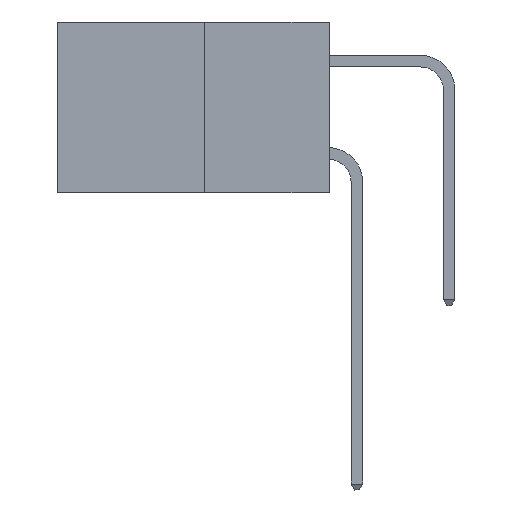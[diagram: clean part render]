
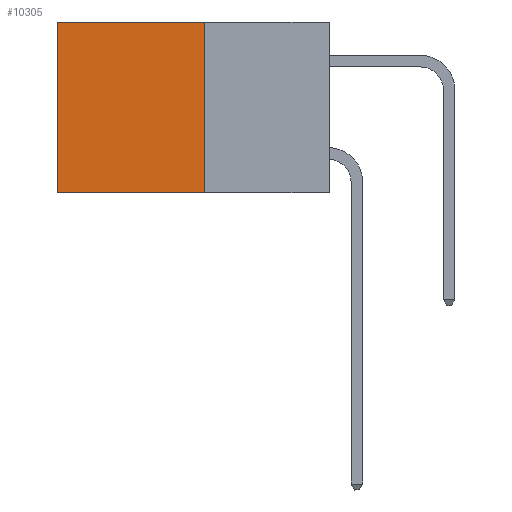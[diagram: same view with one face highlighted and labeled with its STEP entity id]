
A CAD part, left-side view. The second image highlights one B-rep face of the part: STEP entity #10305.
In plain terms, the highlighted planar face has unit normal (-1, 0, 0).
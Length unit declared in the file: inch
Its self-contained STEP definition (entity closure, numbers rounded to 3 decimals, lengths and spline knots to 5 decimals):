
#255 = LINE ( 'NONE', #12976, #3978 ) ;
#1018 = PLANE ( 'NONE',  #6401 ) ;
#1165 = EDGE_CURVE ( 'NONE', #4033, #9187, #13023, .T. ) ;
#1193 = CARTESIAN_POINT ( 'NONE',  ( 0.277, 0.59, 0. ) ) ;
#2083 = FACE_OUTER_BOUND ( 'NONE', #4950, .T. ) ;
#2296 = DIRECTION ( 'NONE',  ( 1., 0., 0. ) ) ;
#3022 = EDGE_CURVE ( 'NONE', #4033, #8451, #11666, .T. ) ;
#3113 = VECTOR ( 'NONE', #9914, 39.37008 ) ;
#3680 = CARTESIAN_POINT ( 'NONE',  ( 0.277, 0.27, 0. ) ) ;
#3850 = DIRECTION ( 'NONE',  ( 0., 1., 0. ) ) ;
#3978 = VECTOR ( 'NONE', #14117, 39.37008 ) ;
#4033 = VERTEX_POINT ( 'NONE', #3680 ) ;
#4950 = EDGE_LOOP ( 'NONE', ( #5924, #10772, #14763, #9836 ) ) ;
#5924 = ORIENTED_EDGE ( 'NONE', *, *, #13153, .T. ) ;
#6401 = AXIS2_PLACEMENT_3D ( 'NONE', #9809, #2296, #11016 ) ;
#8451 = VERTEX_POINT ( 'NONE', #1193 ) ;
#8939 = VECTOR ( 'NONE', #3850, 39.37008 ) ;
#8969 = CARTESIAN_POINT ( 'NONE',  ( 0.277, 0.27, -0.37 ) ) ;
#9187 = VERTEX_POINT ( 'NONE', #8969 ) ;
#9809 = CARTESIAN_POINT ( 'NONE',  ( 0.277, 0.27, -0.37 ) ) ;
#9836 = ORIENTED_EDGE ( 'NONE', *, *, #3022, .T. ) ;
#9914 = DIRECTION ( 'NONE',  ( 0., 0., -1. ) ) ;
#10180 = CARTESIAN_POINT ( 'NONE',  ( 0.277, 0.27, -0.37 ) ) ;
#10305 = ADVANCED_FACE ( 'NONE', ( #2083 ), #1018, .F. ) ;
#10772 = ORIENTED_EDGE ( 'NONE', *, *, #11637, .F. ) ;
#11016 = DIRECTION ( 'NONE',  ( 0., 0., -1. ) ) ;
#11637 = EDGE_CURVE ( 'NONE', #9187, #14274, #12202, .T. ) ;
#11666 = LINE ( 'NONE', #13446, #14506 ) ;
#12202 = LINE ( 'NONE', #14925, #8939 ) ;
#12976 = CARTESIAN_POINT ( 'NONE',  ( 0.277, 0.59, -0.37 ) ) ;
#13023 = LINE ( 'NONE', #10180, #3113 ) ;
#13153 = EDGE_CURVE ( 'NONE', #8451, #14274, #255, .T. ) ;
#13446 = CARTESIAN_POINT ( 'NONE',  ( 0.277, 0.27, 0. ) ) ;
#13876 = CARTESIAN_POINT ( 'NONE',  ( 0.277, 0.59, -0.37 ) ) ;
#14117 = DIRECTION ( 'NONE',  ( 0., 0., -1. ) ) ;
#14274 = VERTEX_POINT ( 'NONE', #13876 ) ;
#14506 = VECTOR ( 'NONE', #14510, 39.37008 ) ;
#14510 = DIRECTION ( 'NONE',  ( 0., 1., 0. ) ) ;
#14763 = ORIENTED_EDGE ( 'NONE', *, *, #1165, .F. ) ;
#14925 = CARTESIAN_POINT ( 'NONE',  ( 0.277, 0.27, -0.37 ) ) ;
